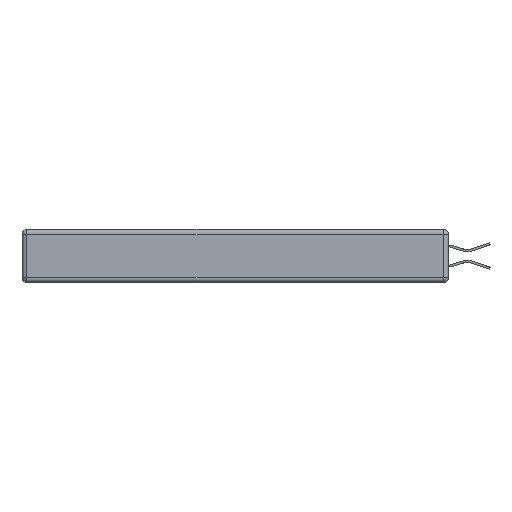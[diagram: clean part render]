
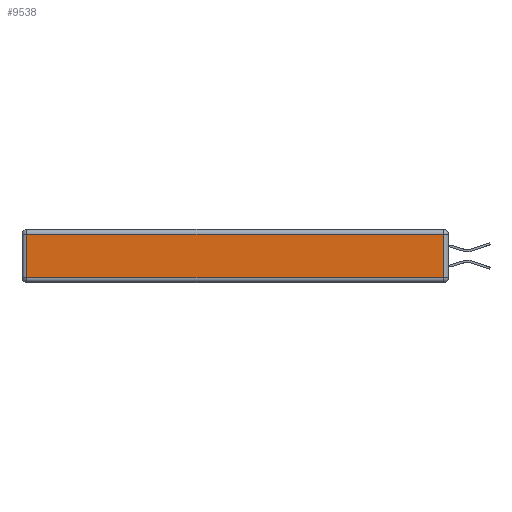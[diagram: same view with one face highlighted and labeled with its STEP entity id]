
A CAD part, left-side view. The second image highlights one B-rep face of the part: STEP entity #9538.
In plain terms, the highlighted planar face has unit normal (-1, 0, 0).
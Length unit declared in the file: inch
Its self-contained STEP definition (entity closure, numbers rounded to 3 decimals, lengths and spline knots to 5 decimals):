
#821 = EDGE_CURVE ( 'NONE', #4083, #6476, #7443, .T. ) ;
#893 = CARTESIAN_POINT ( 'NONE',  ( 0., 0.03, -0.343 ) ) ;
#915 = ORIENTED_EDGE ( 'NONE', *, *, #11415, .T. ) ;
#1364 = DIRECTION ( 'NONE',  ( 0., 0., -1. ) ) ;
#2587 = VERTEX_POINT ( 'NONE', #3569 ) ;
#2826 = EDGE_CURVE ( 'NONE', #2587, #6741, #11708, .T. ) ;
#3131 = CARTESIAN_POINT ( 'NONE',  ( 0., 0.03, -0.03 ) ) ;
#3569 = CARTESIAN_POINT ( 'NONE',  ( 0., 0.03, -0.313 ) ) ;
#4083 = VERTEX_POINT ( 'NONE', #10425 ) ;
#4348 = ORIENTED_EDGE ( 'NONE', *, *, #821, .T. ) ;
#5134 = AXIS2_PLACEMENT_3D ( 'NONE', #14255, #7694, #13027 ) ;
#5632 = ORIENTED_EDGE ( 'NONE', *, *, #2826, .T. ) ;
#5754 = CARTESIAN_POINT ( 'NONE',  ( 0., 0., -0.313 ) ) ;
#5767 = CARTESIAN_POINT ( 'NONE',  ( 0., 2.72, -0.343 ) ) ;
#6396 = FACE_OUTER_BOUND ( 'NONE', #8961, .T. ) ;
#6438 = CARTESIAN_POINT ( 'NONE',  ( 0., 2.72, -0.313 ) ) ;
#6476 = VERTEX_POINT ( 'NONE', #6438 ) ;
#6576 = PLANE ( 'NONE',  #5134 ) ;
#6741 = VERTEX_POINT ( 'NONE', #3131 ) ;
#6863 = VECTOR ( 'NONE', #8627, 39.37008 ) ;
#7443 = LINE ( 'NONE', #5767, #12266 ) ;
#7694 = DIRECTION ( 'NONE',  ( -1., 0., 0. ) ) ;
#7861 = VECTOR ( 'NONE', #10211, 39.37008 ) ;
#8445 = DIRECTION ( 'NONE',  ( 0., 1., 0. ) ) ;
#8625 = ORIENTED_EDGE ( 'NONE', *, *, #14152, .T. ) ;
#8627 = DIRECTION ( 'NONE',  ( 0., 0., 1. ) ) ;
#8961 = EDGE_LOOP ( 'NONE', ( #915, #5632, #8625, #4348 ) ) ;
#9357 = VECTOR ( 'NONE', #8445, 39.37008 ) ;
#9538 = ADVANCED_FACE ( 'NONE', ( #6396 ), #6576, .T. ) ;
#10211 = DIRECTION ( 'NONE',  ( 0., -1., 0. ) ) ;
#10425 = CARTESIAN_POINT ( 'NONE',  ( 0., 2.72, -0.03 ) ) ;
#11155 = LINE ( 'NONE', #5754, #7861 ) ;
#11415 = EDGE_CURVE ( 'NONE', #6476, #2587, #11155, .T. ) ;
#11708 = LINE ( 'NONE', #893, #6863 ) ;
#12266 = VECTOR ( 'NONE', #1364, 39.37008 ) ;
#12843 = CARTESIAN_POINT ( 'NONE',  ( 0., 2.75, -0.03 ) ) ;
#13027 = DIRECTION ( 'NONE',  ( 0., 0., 1. ) ) ;
#13802 = LINE ( 'NONE', #12843, #9357 ) ;
#14152 = EDGE_CURVE ( 'NONE', #6741, #4083, #13802, .T. ) ;
#14255 = CARTESIAN_POINT ( 'NONE',  ( 0., 0., -0.343 ) ) ;
